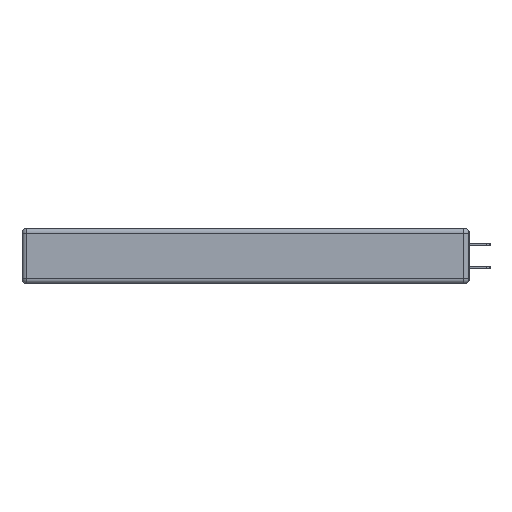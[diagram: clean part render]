
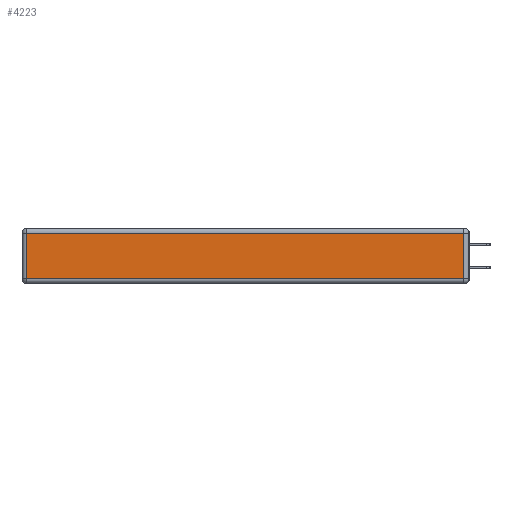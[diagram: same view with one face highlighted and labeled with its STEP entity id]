
A CAD part, left-side view. The second image highlights one B-rep face of the part: STEP entity #4223.
In plain terms, the highlighted planar face has unit normal (-1, 0, 0).
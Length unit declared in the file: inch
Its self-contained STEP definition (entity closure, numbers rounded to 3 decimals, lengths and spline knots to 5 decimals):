
#1451 = EDGE_CURVE ( 'NONE', #25220, #20811, #16101, .T. ) ;
#2365 = VECTOR ( 'NONE', #28459, 39.37008 ) ;
#2666 = ORIENTED_EDGE ( 'NONE', *, *, #14738, .T. ) ;
#3630 = ORIENTED_EDGE ( 'NONE', *, *, #7507, .T. ) ;
#4223 = ADVANCED_FACE ( 'NONE', ( #9014 ), #7753, .T. ) ;
#5301 = VECTOR ( 'NONE', #29290, 39.37008 ) ;
#7507 = EDGE_CURVE ( 'NONE', #13812, #25232, #21759, .T. ) ;
#7753 = PLANE ( 'NONE',  #13272 ) ;
#7953 = DIRECTION ( 'NONE',  ( 0., 0., 1. ) ) ;
#9014 = FACE_OUTER_BOUND ( 'NONE', #28246, .T. ) ;
#9626 = CARTESIAN_POINT ( 'NONE',  ( 0., 2.72, -0.343 ) ) ;
#10088 = CARTESIAN_POINT ( 'NONE',  ( 0., 0., -0.343 ) ) ;
#10526 = CARTESIAN_POINT ( 'NONE',  ( 0., 2.75, -0.03 ) ) ;
#11889 = EDGE_CURVE ( 'NONE', #20811, #13812, #27297, .T. ) ;
#12510 = CARTESIAN_POINT ( 'NONE',  ( 0., 0., -0.313 ) ) ;
#12564 = DIRECTION ( 'NONE',  ( 0., 0., 1. ) ) ;
#13269 = CARTESIAN_POINT ( 'NONE',  ( 0., 2.72, -0.03 ) ) ;
#13272 = AXIS2_PLACEMENT_3D ( 'NONE', #10088, #21641, #7953 ) ;
#13560 = VECTOR ( 'NONE', #12564, 39.37008 ) ;
#13812 = VERTEX_POINT ( 'NONE', #13269 ) ;
#14738 = EDGE_CURVE ( 'NONE', #25232, #25220, #25349, .T. ) ;
#16101 = LINE ( 'NONE', #17610, #13560 ) ;
#17610 = CARTESIAN_POINT ( 'NONE',  ( 0., 0.03, -0.343 ) ) ;
#20040 = CARTESIAN_POINT ( 'NONE',  ( 0., 0.03, -0.03 ) ) ;
#20811 = VERTEX_POINT ( 'NONE', #20040 ) ;
#21641 = DIRECTION ( 'NONE',  ( -1., 0., 0. ) ) ;
#21759 = LINE ( 'NONE', #9626, #2365 ) ;
#21764 = DIRECTION ( 'NONE',  ( 0., -1., 0. ) ) ;
#22716 = ORIENTED_EDGE ( 'NONE', *, *, #11889, .T. ) ;
#24641 = CARTESIAN_POINT ( 'NONE',  ( 0., 2.72, -0.313 ) ) ;
#25191 = ORIENTED_EDGE ( 'NONE', *, *, #1451, .T. ) ;
#25220 = VERTEX_POINT ( 'NONE', #29292 ) ;
#25232 = VERTEX_POINT ( 'NONE', #24641 ) ;
#25349 = LINE ( 'NONE', #12510, #26784 ) ;
#26784 = VECTOR ( 'NONE', #21764, 39.37008 ) ;
#27297 = LINE ( 'NONE', #10526, #5301 ) ;
#28246 = EDGE_LOOP ( 'NONE', ( #2666, #25191, #22716, #3630 ) ) ;
#28459 = DIRECTION ( 'NONE',  ( 0., 0., -1. ) ) ;
#29290 = DIRECTION ( 'NONE',  ( 0., 1., 0. ) ) ;
#29292 = CARTESIAN_POINT ( 'NONE',  ( 0., 0.03, -0.313 ) ) ;
